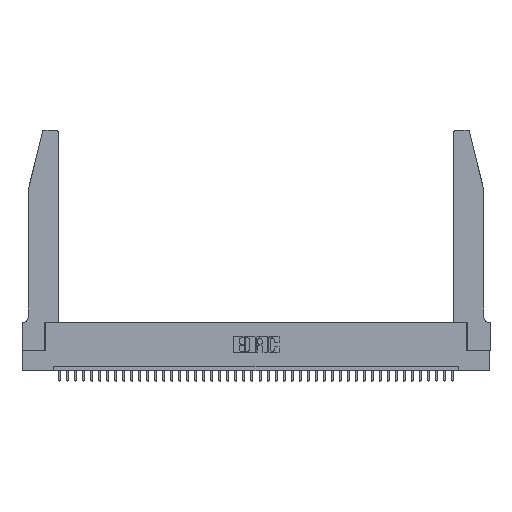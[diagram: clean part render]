
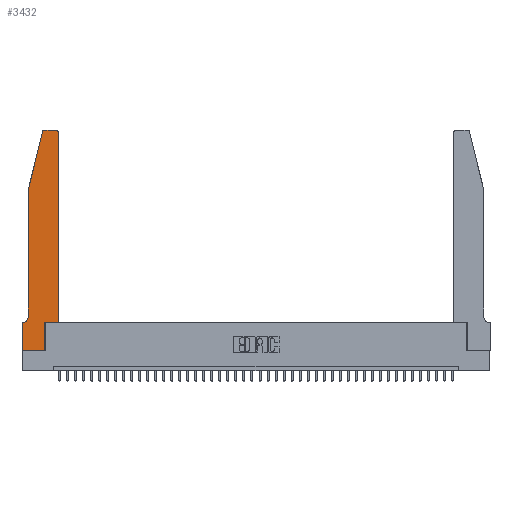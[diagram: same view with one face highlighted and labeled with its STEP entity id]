
A CAD part, top view. The second image highlights one B-rep face of the part: STEP entity #3432.
In plain terms, the highlighted planar face has unit normal (0, 0, 1).
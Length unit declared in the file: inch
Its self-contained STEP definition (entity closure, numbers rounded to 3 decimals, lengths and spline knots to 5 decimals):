
#85 = EDGE_CURVE ( 'NONE', #1815, #1834, #33126, .T. ) ;
#335 = CARTESIAN_POINT ( 'NONE',  ( 0.0755, 0.35, 0.37 ) ) ;
#427 = ORIENTED_EDGE ( 'NONE', *, *, #1960, .T. ) ;
#656 = PLANE ( 'NONE',  #5224 ) ;
#688 = VERTEX_POINT ( 'NONE', #26551 ) ;
#792 = DIRECTION ( 'NONE',  ( -0.239, -0.971, 0. ) ) ;
#924 = CARTESIAN_POINT ( 'NONE',  ( 0.2605, 2.75, 0.37 ) ) ;
#939 = DIRECTION ( 'NONE',  ( 0., 0., 1. ) ) ;
#949 = CIRCLE ( 'NONE', #13699, 0.07 ) ;
#1815 = VERTEX_POINT ( 'NONE', #35329 ) ;
#1834 = VERTEX_POINT ( 'NONE', #32023 ) ;
#1960 = EDGE_CURVE ( 'NONE', #2627, #32063, #8037, .T. ) ;
#2026 = EDGE_CURVE ( 'NONE', #3539, #688, #6981, .T. ) ;
#2364 = VECTOR ( 'NONE', #28816, 39.37008 ) ;
#2627 = VERTEX_POINT ( 'NONE', #21619 ) ;
#3432 = ADVANCED_FACE ( 'NONE', ( #35258 ), #656, .T. ) ;
#3539 = VERTEX_POINT ( 'NONE', #27748 ) ;
#5224 = AXIS2_PLACEMENT_3D ( 'NONE', #39032, #939, #19974 ) ;
#5766 = CARTESIAN_POINT ( 'NONE',  ( 0.4505, 0.35, 0.37 ) ) ;
#5984 = CARTESIAN_POINT ( 'NONE',  ( 0.4205, 2.72, 0.37 ) ) ;
#6981 = LINE ( 'NONE', #924, #39983 ) ;
#7093 = CARTESIAN_POINT ( 'NONE',  ( 0.0755, 2., 0.37 ) ) ;
#7532 = VERTEX_POINT ( 'NONE', #23754 ) ;
#7926 = VERTEX_POINT ( 'NONE', #18126 ) ;
#8037 = LINE ( 'NONE', #7093, #35906 ) ;
#8123 = CARTESIAN_POINT ( 'NONE',  ( 0.0055, 0.42, 0.37 ) ) ;
#8529 = ORIENTED_EDGE ( 'NONE', *, *, #23659, .T. ) ;
#9527 = CIRCLE ( 'NONE', #33027, 0.03 ) ;
#9553 = DIRECTION ( 'NONE',  ( 0., -1., 0. ) ) ;
#10593 = EDGE_CURVE ( 'NONE', #1834, #16146, #18394, .T. ) ;
#11189 = VECTOR ( 'NONE', #24754, 39.37008 ) ;
#11606 = ORIENTED_EDGE ( 'NONE', *, *, #10593, .T. ) ;
#12413 = DIRECTION ( 'NONE',  ( 1., 0., 0. ) ) ;
#13274 = VECTOR ( 'NONE', #9553, 39.37008 ) ;
#13695 = DIRECTION ( 'NONE',  ( 1., 0., 0. ) ) ;
#13699 = AXIS2_PLACEMENT_3D ( 'NONE', #8123, #34190, #18054 ) ;
#13812 = EDGE_LOOP ( 'NONE', ( #20190, #38198, #427, #39843, #20051, #28624, #25157, #8529, #20889, #17574, #11606, #23076 ) ) ;
#14454 = LINE ( 'NONE', #32346, #16397 ) ;
#15053 = DIRECTION ( 'NONE',  ( 0., 0., 1. ) ) ;
#15150 = CARTESIAN_POINT ( 'NONE',  ( 0.0055, 0.35, 0.37 ) ) ;
#15427 = VERTEX_POINT ( 'NONE', #15697 ) ;
#15520 = CIRCLE ( 'NONE', #37245, 0.03 ) ;
#15697 = CARTESIAN_POINT ( 'NONE',  ( 0., 0., 0.37 ) ) ;
#15954 = CARTESIAN_POINT ( 'NONE',  ( 0.2865, 0.35, 0.37 ) ) ;
#16060 = VERTEX_POINT ( 'NONE', #36666 ) ;
#16146 = VERTEX_POINT ( 'NONE', #18167 ) ;
#16397 = VECTOR ( 'NONE', #13695, 39.37008 ) ;
#17020 = DIRECTION ( 'NONE',  ( -1., 0., 0. ) ) ;
#17574 = ORIENTED_EDGE ( 'NONE', *, *, #85, .T. ) ;
#17843 = DIRECTION ( 'NONE',  ( 0., -1., 0. ) ) ;
#18054 = DIRECTION ( 'NONE',  ( -1., 0., 0. ) ) ;
#18126 = CARTESIAN_POINT ( 'NONE',  ( 0.2865, 0., 0.37 ) ) ;
#18167 = CARTESIAN_POINT ( 'NONE',  ( 0.4505, 2.72, 0.37 ) ) ;
#18364 = LINE ( 'NONE', #15954, #2364 ) ;
#18394 = LINE ( 'NONE', #23004, #18884 ) ;
#18637 = CARTESIAN_POINT ( 'NONE',  ( 0.284, 2.72, 0.37 ) ) ;
#18884 = VECTOR ( 'NONE', #23581, 39.37008 ) ;
#19974 = DIRECTION ( 'NONE',  ( 1., 0., 0. ) ) ;
#20051 = ORIENTED_EDGE ( 'NONE', *, *, #22717, .T. ) ;
#20190 = ORIENTED_EDGE ( 'NONE', *, *, #2026, .T. ) ;
#20889 = ORIENTED_EDGE ( 'NONE', *, *, #40842, .T. ) ;
#21619 = CARTESIAN_POINT ( 'NONE',  ( 0.25487, 2.72718, 0.37 ) ) ;
#22305 = CARTESIAN_POINT ( 'NONE',  ( 0., 0., 0.37 ) ) ;
#22703 = DIRECTION ( 'NONE',  ( -1., 0., 0. ) ) ;
#22717 = EDGE_CURVE ( 'NONE', #7532, #22761, #949, .T. ) ;
#22761 = VERTEX_POINT ( 'NONE', #15150 ) ;
#23004 = CARTESIAN_POINT ( 'NONE',  ( 0.4505, 0.35, 0.37 ) ) ;
#23076 = ORIENTED_EDGE ( 'NONE', *, *, #23220, .T. ) ;
#23220 = EDGE_CURVE ( 'NONE', #16146, #3539, #15520, .T. ) ;
#23581 = DIRECTION ( 'NONE',  ( 0., 1., 0. ) ) ;
#23659 = EDGE_CURVE ( 'NONE', #15427, #7926, #14454, .T. ) ;
#23754 = CARTESIAN_POINT ( 'NONE',  ( 0.0755, 0.42, 0.37 ) ) ;
#24720 = EDGE_CURVE ( 'NONE', #22761, #16060, #36221, .T. ) ;
#24754 = DIRECTION ( 'NONE',  ( 1., 0., 0. ) ) ;
#25157 = ORIENTED_EDGE ( 'NONE', *, *, #35415, .T. ) ;
#26551 = CARTESIAN_POINT ( 'NONE',  ( 0.284, 2.75, 0.37 ) ) ;
#27583 = VECTOR ( 'NONE', #17843, 39.37008 ) ;
#27748 = CARTESIAN_POINT ( 'NONE',  ( 0.4205, 2.75, 0.37 ) ) ;
#28270 = DIRECTION ( 'NONE',  ( 0., 0., 1. ) ) ;
#28624 = ORIENTED_EDGE ( 'NONE', *, *, #24720, .T. ) ;
#28816 = DIRECTION ( 'NONE',  ( 0., 1., 0. ) ) ;
#28949 = EDGE_CURVE ( 'NONE', #688, #2627, #9527, .T. ) ;
#31265 = LINE ( 'NONE', #22305, #13274 ) ;
#32023 = CARTESIAN_POINT ( 'NONE',  ( 0.4505, 0.35, 0.37 ) ) ;
#32063 = VERTEX_POINT ( 'NONE', #40210 ) ;
#32303 = EDGE_CURVE ( 'NONE', #32063, #7532, #39028, .T. ) ;
#32346 = CARTESIAN_POINT ( 'NONE',  ( 0., 0., 0.37 ) ) ;
#33027 = AXIS2_PLACEMENT_3D ( 'NONE', #18637, #15053, #37441 ) ;
#33126 = LINE ( 'NONE', #5766, #11189 ) ;
#34190 = DIRECTION ( 'NONE',  ( 0., 0., -1. ) ) ;
#35258 = FACE_OUTER_BOUND ( 'NONE', #13812, .T. ) ;
#35329 = CARTESIAN_POINT ( 'NONE',  ( 0.2865, 0.35, 0.37 ) ) ;
#35415 = EDGE_CURVE ( 'NONE', #16060, #15427, #31265, .T. ) ;
#35906 = VECTOR ( 'NONE', #792, 39.37008 ) ;
#36221 = LINE ( 'NONE', #335, #37283 ) ;
#36666 = CARTESIAN_POINT ( 'NONE',  ( 0., 0.35, 0.37 ) ) ;
#37071 = CARTESIAN_POINT ( 'NONE',  ( 0.0755, 2., 0.37 ) ) ;
#37245 = AXIS2_PLACEMENT_3D ( 'NONE', #5984, #28270, #12413 ) ;
#37283 = VECTOR ( 'NONE', #22703, 39.37008 ) ;
#37441 = DIRECTION ( 'NONE',  ( 1., 0., 0. ) ) ;
#38198 = ORIENTED_EDGE ( 'NONE', *, *, #28949, .T. ) ;
#39028 = LINE ( 'NONE', #37071, #27583 ) ;
#39032 = CARTESIAN_POINT ( 'NONE',  ( 0., 0.35, 0.37 ) ) ;
#39843 = ORIENTED_EDGE ( 'NONE', *, *, #32303, .T. ) ;
#39983 = VECTOR ( 'NONE', #17020, 39.37008 ) ;
#40210 = CARTESIAN_POINT ( 'NONE',  ( 0.0755, 2., 0.37 ) ) ;
#40842 = EDGE_CURVE ( 'NONE', #7926, #1815, #18364, .T. ) ;
